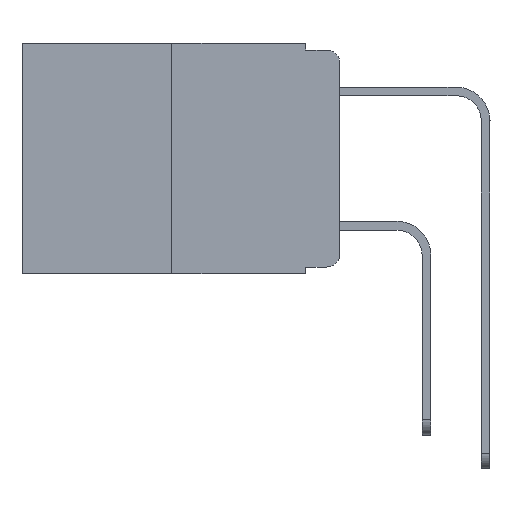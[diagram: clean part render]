
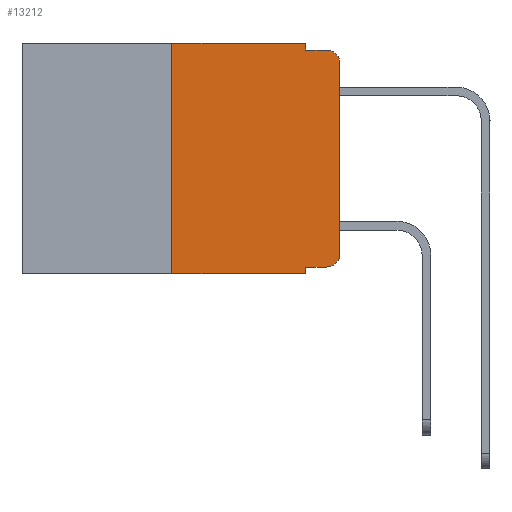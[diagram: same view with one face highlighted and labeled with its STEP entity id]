
A CAD part, left-side view. The second image highlights one B-rep face of the part: STEP entity #13212.
In plain terms, the highlighted planar face has unit normal (-1, 0, 0).
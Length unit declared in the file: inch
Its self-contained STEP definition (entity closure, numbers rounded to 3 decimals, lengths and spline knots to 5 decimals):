
#161 = VERTEX_POINT ( 'NONE', #22908 ) ;
#932 = ORIENTED_EDGE ( 'NONE', *, *, #11022, .F. ) ;
#1152 = DIRECTION ( 'NONE',  ( 1., 0., 0. ) ) ;
#1165 = CARTESIAN_POINT ( 'NONE',  ( 0., 0.473, -0.343 ) ) ;
#1169 = DIRECTION ( 'NONE',  ( 0., 0., -1. ) ) ;
#1268 = CARTESIAN_POINT ( 'NONE',  ( 0., 0.25, 0. ) ) ;
#1564 = LINE ( 'NONE', #2716, #20579 ) ;
#2051 = EDGE_CURVE ( 'NONE', #10123, #8792, #7851, .T. ) ;
#2122 = DIRECTION ( 'NONE',  ( 0., 0., 1. ) ) ;
#2716 = CARTESIAN_POINT ( 'NONE',  ( 0., 0., 0. ) ) ;
#3181 = ORIENTED_EDGE ( 'NONE', *, *, #2051, .T. ) ;
#3200 = CIRCLE ( 'NONE', #15972, 0.02 ) ;
#3296 = CARTESIAN_POINT ( 'NONE',  ( 0., 0.051, 0. ) ) ;
#4084 = EDGE_CURVE ( 'NONE', #9461, #19728, #16903, .T. ) ;
#4734 = EDGE_CURVE ( 'NONE', #161, #10123, #9821, .T. ) ;
#5280 = VECTOR ( 'NONE', #20955, 39.37008 ) ;
#5567 = ORIENTED_EDGE ( 'NONE', *, *, #15015, .F. ) ;
#5618 = VECTOR ( 'NONE', #21842, 39.37008 ) ;
#6672 = DIRECTION ( 'NONE',  ( 0., 0., 1. ) ) ;
#6801 = CARTESIAN_POINT ( 'NONE',  ( 0., 0.02, -0.333 ) ) ;
#6940 = CARTESIAN_POINT ( 'NONE',  ( 0., 0.051, -0.01 ) ) ;
#7324 = EDGE_CURVE ( 'NONE', #161, #19728, #10028, .T. ) ;
#7737 = ORIENTED_EDGE ( 'NONE', *, *, #4084, .T. ) ;
#7851 = CIRCLE ( 'NONE', #8394, 0.02 ) ;
#8359 = LINE ( 'NONE', #13759, #18311 ) ;
#8394 = AXIS2_PLACEMENT_3D ( 'NONE', #8502, #13557, #13912 ) ;
#8502 = CARTESIAN_POINT ( 'NONE',  ( 0., 0.02, -0.313 ) ) ;
#8614 = EDGE_CURVE ( 'NONE', #9461, #12592, #8359, .T. ) ;
#8750 = CARTESIAN_POINT ( 'NONE',  ( 0., 0.25, -0.343 ) ) ;
#8792 = VERTEX_POINT ( 'NONE', #23453 ) ;
#9218 = ORIENTED_EDGE ( 'NONE', *, *, #8614, .F. ) ;
#9461 = VERTEX_POINT ( 'NONE', #8750 ) ;
#9703 = CARTESIAN_POINT ( 'NONE',  ( 0., 0.02, -0.01 ) ) ;
#9705 = VECTOR ( 'NONE', #19250, 39.37008 ) ;
#9789 = ORIENTED_EDGE ( 'NONE', *, *, #17438, .T. ) ;
#9821 = LINE ( 'NONE', #14131, #5280 ) ;
#9924 = EDGE_CURVE ( 'NONE', #20595, #14847, #15153, .T. ) ;
#9967 = VECTOR ( 'NONE', #23769, 39.37008 ) ;
#10003 = CARTESIAN_POINT ( 'NONE',  ( 0., 0.473, 0. ) ) ;
#10028 = LINE ( 'NONE', #3296, #14487 ) ;
#10123 = VERTEX_POINT ( 'NONE', #6801 ) ;
#10404 = ORIENTED_EDGE ( 'NONE', *, *, #16235, .T. ) ;
#11022 = EDGE_CURVE ( 'NONE', #12592, #20595, #14213, .T. ) ;
#11367 = ORIENTED_EDGE ( 'NONE', *, *, #7324, .F. ) ;
#11570 = VERTEX_POINT ( 'NONE', #9703 ) ;
#11967 = CARTESIAN_POINT ( 'NONE',  ( 0., 0.051, 0. ) ) ;
#12266 = CARTESIAN_POINT ( 'NONE',  ( 0., 0.051, -0.01 ) ) ;
#12592 = VERTEX_POINT ( 'NONE', #1268 ) ;
#12639 = FACE_OUTER_BOUND ( 'NONE', #24138, .T. ) ;
#12866 = DIRECTION ( 'NONE',  ( -1., 0., 0. ) ) ;
#13212 = ADVANCED_FACE ( 'NONE', ( #12639 ), #23865, .F. ) ;
#13557 = DIRECTION ( 'NONE',  ( -1., 0., 0. ) ) ;
#13759 = CARTESIAN_POINT ( 'NONE',  ( 0., 0.25, 0. ) ) ;
#13912 = DIRECTION ( 'NONE',  ( 0., 0., -1. ) ) ;
#14131 = CARTESIAN_POINT ( 'NONE',  ( 0., 0.051, -0.333 ) ) ;
#14213 = LINE ( 'NONE', #10003, #9705 ) ;
#14349 = ORIENTED_EDGE ( 'NONE', *, *, #4734, .T. ) ;
#14487 = VECTOR ( 'NONE', #14840, 39.37008 ) ;
#14719 = DIRECTION ( 'NONE',  ( 0., 0., -1. ) ) ;
#14840 = DIRECTION ( 'NONE',  ( 0., 0., -1. ) ) ;
#14847 = VERTEX_POINT ( 'NONE', #12266 ) ;
#15015 = EDGE_CURVE ( 'NONE', #14847, #11570, #15016, .T. ) ;
#15016 = LINE ( 'NONE', #6940, #9967 ) ;
#15153 = LINE ( 'NONE', #11967, #22603 ) ;
#15379 = CARTESIAN_POINT ( 'NONE',  ( 0., 0.051, 0. ) ) ;
#15972 = AXIS2_PLACEMENT_3D ( 'NONE', #23874, #12866, #1169 ) ;
#16235 = EDGE_CURVE ( 'NONE', #23375, #11570, #3200, .T. ) ;
#16903 = LINE ( 'NONE', #1165, #5618 ) ;
#17438 = EDGE_CURVE ( 'NONE', #8792, #23375, #1564, .T. ) ;
#17524 = DIRECTION ( 'NONE',  ( 0., 0., -1. ) ) ;
#18271 = CARTESIAN_POINT ( 'NONE',  ( 0., 0.473, 0. ) ) ;
#18311 = VECTOR ( 'NONE', #2122, 39.37008 ) ;
#19250 = DIRECTION ( 'NONE',  ( 0., -1., 0. ) ) ;
#19728 = VERTEX_POINT ( 'NONE', #23589 ) ;
#20579 = VECTOR ( 'NONE', #6672, 39.37008 ) ;
#20595 = VERTEX_POINT ( 'NONE', #15379 ) ;
#20955 = DIRECTION ( 'NONE',  ( 0., -1., 0. ) ) ;
#21464 = CARTESIAN_POINT ( 'NONE',  ( 0., 0., -0.03 ) ) ;
#21842 = DIRECTION ( 'NONE',  ( 0., -1., 0. ) ) ;
#22536 = AXIS2_PLACEMENT_3D ( 'NONE', #18271, #1152, #14719 ) ;
#22603 = VECTOR ( 'NONE', #17524, 39.37008 ) ;
#22631 = ORIENTED_EDGE ( 'NONE', *, *, #9924, .F. ) ;
#22908 = CARTESIAN_POINT ( 'NONE',  ( 0., 0.051, -0.333 ) ) ;
#23375 = VERTEX_POINT ( 'NONE', #21464 ) ;
#23453 = CARTESIAN_POINT ( 'NONE',  ( 0., 0., -0.313 ) ) ;
#23589 = CARTESIAN_POINT ( 'NONE',  ( 0., 0.051, -0.343 ) ) ;
#23769 = DIRECTION ( 'NONE',  ( 0., -1., 0. ) ) ;
#23865 = PLANE ( 'NONE',  #22536 ) ;
#23874 = CARTESIAN_POINT ( 'NONE',  ( 0., 0.02, -0.03 ) ) ;
#24138 = EDGE_LOOP ( 'NONE', ( #9789, #10404, #5567, #22631, #932, #9218, #7737, #11367, #14349, #3181 ) ) ;
